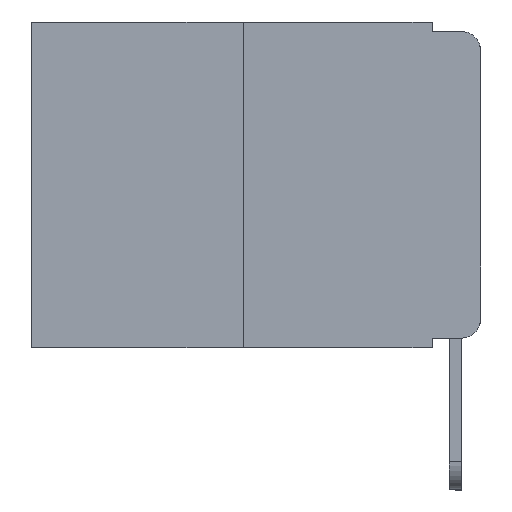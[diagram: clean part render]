
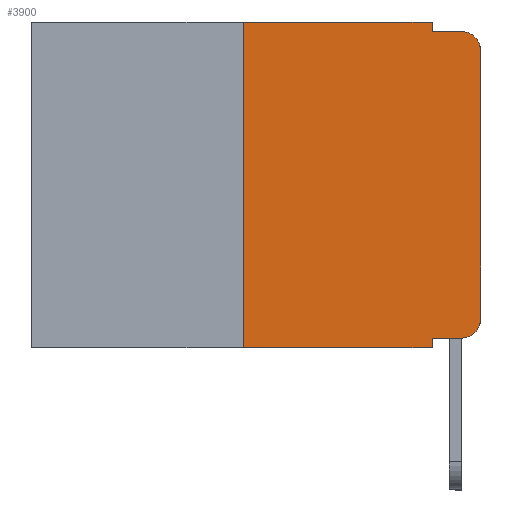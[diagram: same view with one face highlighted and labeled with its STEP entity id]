
A CAD part, left-side view. The second image highlights one B-rep face of the part: STEP entity #3900.
In plain terms, the highlighted planar face has unit normal (-1, 0, 0).
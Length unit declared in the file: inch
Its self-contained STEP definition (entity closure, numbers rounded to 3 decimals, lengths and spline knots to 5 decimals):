
#58 = EDGE_LOOP ( 'NONE', ( #3099, #9131, #13181, #7570, #7478, #7816, #14737, #11152, #10981, #4956 ) ) ;
#293 = CARTESIAN_POINT ( 'NONE',  ( 0., 0., -0.313 ) ) ;
#334 = AXIS2_PLACEMENT_3D ( 'NONE', #14117, #11383, #7558 ) ;
#673 = EDGE_CURVE ( 'NONE', #839, #11508, #6270, .T. ) ;
#798 = VERTEX_POINT ( 'NONE', #917 ) ;
#839 = VERTEX_POINT ( 'NONE', #293 ) ;
#917 = CARTESIAN_POINT ( 'NONE',  ( 0., 0.25, 0. ) ) ;
#1025 = EDGE_CURVE ( 'NONE', #3215, #7368, #13606, .T. ) ;
#1052 = DIRECTION ( 'NONE',  ( 0., -1., 0. ) ) ;
#1236 = DIRECTION ( 'NONE',  ( -1., 0., 0. ) ) ;
#1411 = CARTESIAN_POINT ( 'NONE',  ( 0., 0.02, -0.313 ) ) ;
#2137 = CARTESIAN_POINT ( 'NONE',  ( 0., 0.051, 0. ) ) ;
#2472 = DIRECTION ( 'NONE',  ( -1., 0., 0. ) ) ;
#2868 = EDGE_CURVE ( 'NONE', #5488, #5094, #12473, .T. ) ;
#2884 = VECTOR ( 'NONE', #10198, 39.37008 ) ;
#3099 = ORIENTED_EDGE ( 'NONE', *, *, #673, .T. ) ;
#3215 = VERTEX_POINT ( 'NONE', #11415 ) ;
#3319 = EDGE_CURVE ( 'NONE', #11318, #4909, #9219, .T. ) ;
#3520 = CARTESIAN_POINT ( 'NONE',  ( 0., 0.051, -0.333 ) ) ;
#3597 = CARTESIAN_POINT ( 'NONE',  ( 0., 0.051, 0. ) ) ;
#3842 = VECTOR ( 'NONE', #9036, 39.37008 ) ;
#3853 = CARTESIAN_POINT ( 'NONE',  ( 0., 0.25, -0.343 ) ) ;
#3900 = ADVANCED_FACE ( 'NONE', ( #6192 ), #15413, .F. ) ;
#4305 = LINE ( 'NONE', #14794, #16656 ) ;
#4445 = EDGE_CURVE ( 'NONE', #798, #7244, #14349, .T. ) ;
#4502 = CARTESIAN_POINT ( 'NONE',  ( 0., 0.051, -0.343 ) ) ;
#4909 = VERTEX_POINT ( 'NONE', #4502 ) ;
#4956 = ORIENTED_EDGE ( 'NONE', *, *, #10861, .T. ) ;
#5043 = CARTESIAN_POINT ( 'NONE',  ( 0., 0.051, -0.333 ) ) ;
#5094 = VERTEX_POINT ( 'NONE', #5249 ) ;
#5249 = CARTESIAN_POINT ( 'NONE',  ( 0., 0.02, -0.333 ) ) ;
#5488 = VERTEX_POINT ( 'NONE', #3520 ) ;
#5843 = CARTESIAN_POINT ( 'NONE',  ( 0., 0.051, -0.01 ) ) ;
#6192 = FACE_OUTER_BOUND ( 'NONE', #58, .T. ) ;
#6270 = LINE ( 'NONE', #10182, #8848 ) ;
#7244 = VERTEX_POINT ( 'NONE', #3597 ) ;
#7368 = VERTEX_POINT ( 'NONE', #9488 ) ;
#7411 = CIRCLE ( 'NONE', #16663, 0.02 ) ;
#7478 = ORIENTED_EDGE ( 'NONE', *, *, #4445, .F. ) ;
#7558 = DIRECTION ( 'NONE',  ( 0., 0., -1. ) ) ;
#7570 = ORIENTED_EDGE ( 'NONE', *, *, #14496, .F. ) ;
#7816 = ORIENTED_EDGE ( 'NONE', *, *, #9242, .F. ) ;
#7867 = DIRECTION ( 'NONE',  ( 0., -1., 0. ) ) ;
#8848 = VECTOR ( 'NONE', #15417, 39.37008 ) ;
#9036 = DIRECTION ( 'NONE',  ( 0., -1., 0. ) ) ;
#9131 = ORIENTED_EDGE ( 'NONE', *, *, #11930, .T. ) ;
#9219 = LINE ( 'NONE', #10389, #3842 ) ;
#9242 = EDGE_CURVE ( 'NONE', #11318, #798, #4305, .T. ) ;
#9488 = CARTESIAN_POINT ( 'NONE',  ( 0., 0.02, -0.01 ) ) ;
#10163 = DIRECTION ( 'NONE',  ( 0., 0., -1. ) ) ;
#10182 = CARTESIAN_POINT ( 'NONE',  ( 0., 0., 0. ) ) ;
#10198 = DIRECTION ( 'NONE',  ( 0., 0., -1. ) ) ;
#10389 = CARTESIAN_POINT ( 'NONE',  ( 0., 0.473, -0.343 ) ) ;
#10759 = CARTESIAN_POINT ( 'NONE',  ( 0., 0.473, 0. ) ) ;
#10861 = EDGE_CURVE ( 'NONE', #5094, #839, #7411, .T. ) ;
#10981 = ORIENTED_EDGE ( 'NONE', *, *, #2868, .T. ) ;
#11152 = ORIENTED_EDGE ( 'NONE', *, *, #13532, .F. ) ;
#11318 = VERTEX_POINT ( 'NONE', #3853 ) ;
#11383 = DIRECTION ( 'NONE',  ( 1., 0., 0. ) ) ;
#11415 = CARTESIAN_POINT ( 'NONE',  ( 0., 0.051, -0.01 ) ) ;
#11508 = VERTEX_POINT ( 'NONE', #14335 ) ;
#11516 = AXIS2_PLACEMENT_3D ( 'NONE', #14147, #2472, #11670 ) ;
#11557 = DIRECTION ( 'NONE',  ( 0., 0., -1. ) ) ;
#11558 = LINE ( 'NONE', #2137, #2884 ) ;
#11560 = VECTOR ( 'NONE', #7867, 39.37008 ) ;
#11650 = LINE ( 'NONE', #14130, #15135 ) ;
#11670 = DIRECTION ( 'NONE',  ( 0., 0., -1. ) ) ;
#11930 = EDGE_CURVE ( 'NONE', #11508, #7368, #15350, .T. ) ;
#12473 = LINE ( 'NONE', #5043, #13887 ) ;
#13181 = ORIENTED_EDGE ( 'NONE', *, *, #1025, .F. ) ;
#13532 = EDGE_CURVE ( 'NONE', #5488, #4909, #11650, .T. ) ;
#13606 = LINE ( 'NONE', #5843, #14614 ) ;
#13887 = VECTOR ( 'NONE', #1052, 39.37008 ) ;
#14117 = CARTESIAN_POINT ( 'NONE',  ( 0., 0.473, 0. ) ) ;
#14130 = CARTESIAN_POINT ( 'NONE',  ( 0., 0.051, 0. ) ) ;
#14147 = CARTESIAN_POINT ( 'NONE',  ( 0., 0.02, -0.03 ) ) ;
#14335 = CARTESIAN_POINT ( 'NONE',  ( 0., 0., -0.03 ) ) ;
#14349 = LINE ( 'NONE', #10759, #11560 ) ;
#14496 = EDGE_CURVE ( 'NONE', #7244, #3215, #11558, .T. ) ;
#14614 = VECTOR ( 'NONE', #14796, 39.37008 ) ;
#14737 = ORIENTED_EDGE ( 'NONE', *, *, #3319, .T. ) ;
#14794 = CARTESIAN_POINT ( 'NONE',  ( 0., 0.25, 0. ) ) ;
#14796 = DIRECTION ( 'NONE',  ( 0., -1., 0. ) ) ;
#15135 = VECTOR ( 'NONE', #11557, 39.37008 ) ;
#15350 = CIRCLE ( 'NONE', #11516, 0.02 ) ;
#15413 = PLANE ( 'NONE',  #334 ) ;
#15417 = DIRECTION ( 'NONE',  ( 0., 0., 1. ) ) ;
#15822 = DIRECTION ( 'NONE',  ( 0., 0., 1. ) ) ;
#16656 = VECTOR ( 'NONE', #15822, 39.37008 ) ;
#16663 = AXIS2_PLACEMENT_3D ( 'NONE', #1411, #1236, #10163 ) ;
